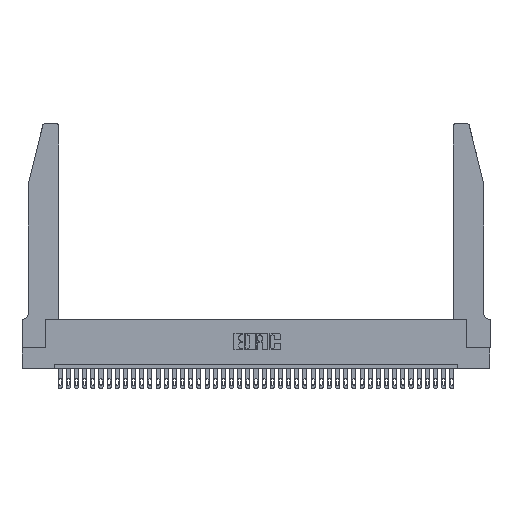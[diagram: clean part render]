
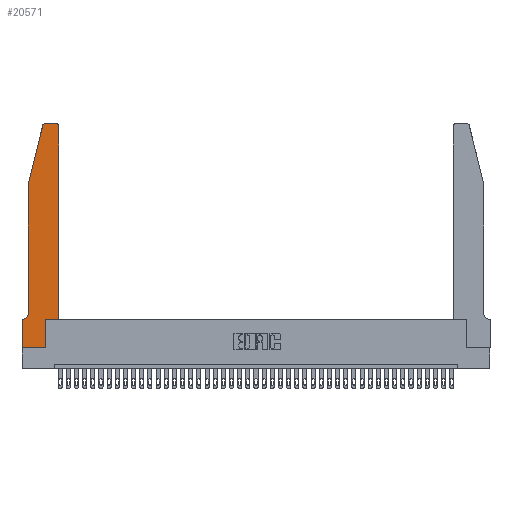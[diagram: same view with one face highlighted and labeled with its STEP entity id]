
A CAD part, top view. The second image highlights one B-rep face of the part: STEP entity #20571.
In plain terms, the highlighted planar face has unit normal (0, 0, 1).
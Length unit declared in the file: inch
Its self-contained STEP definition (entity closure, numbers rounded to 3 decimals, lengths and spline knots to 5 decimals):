
#748 = ORIENTED_EDGE ( 'NONE', *, *, #4426, .T. ) ;
#817 = CARTESIAN_POINT ( 'NONE',  ( 0., 0., 0.37 ) ) ;
#852 = CARTESIAN_POINT ( 'NONE',  ( 0.4505, 0.35, 0.37 ) ) ;
#2289 = EDGE_CURVE ( 'NONE', #5281, #23859, #35067, .T. ) ;
#2867 = CARTESIAN_POINT ( 'NONE',  ( 0.284, 2.75, 0.37 ) ) ;
#3310 = VERTEX_POINT ( 'NONE', #32495 ) ;
#3623 = ORIENTED_EDGE ( 'NONE', *, *, #15255, .T. ) ;
#4426 = EDGE_CURVE ( 'NONE', #23859, #28531, #38317, .T. ) ;
#4523 = ORIENTED_EDGE ( 'NONE', *, *, #11093, .T. ) ;
#4925 = CARTESIAN_POINT ( 'NONE',  ( 0.4505, 0.35, 0.37 ) ) ;
#5281 = VERTEX_POINT ( 'NONE', #11963 ) ;
#5497 = VECTOR ( 'NONE', #39583, 39.37008 ) ;
#5569 = AXIS2_PLACEMENT_3D ( 'NONE', #24513, #27933, #27670 ) ;
#5633 = CARTESIAN_POINT ( 'NONE',  ( 0.4505, 2.72, 0.37 ) ) ;
#5838 = CARTESIAN_POINT ( 'NONE',  ( 0.0055, 0.42, 0.37 ) ) ;
#6523 = CARTESIAN_POINT ( 'NONE',  ( 0.0755, 0.42, 0.37 ) ) ;
#6568 = DIRECTION ( 'NONE',  ( 0., 0., 1. ) ) ;
#6825 = CARTESIAN_POINT ( 'NONE',  ( 0.4205, 2.72, 0.37 ) ) ;
#7433 = EDGE_CURVE ( 'NONE', #28531, #3310, #31796, .T. ) ;
#8090 = DIRECTION ( 'NONE',  ( 1., 0., 0. ) ) ;
#8739 = ORIENTED_EDGE ( 'NONE', *, *, #37533, .T. ) ;
#8813 = ORIENTED_EDGE ( 'NONE', *, *, #30957, .T. ) ;
#8863 = VECTOR ( 'NONE', #28510, 39.37008 ) ;
#8912 = VECTOR ( 'NONE', #32799, 39.37008 ) ;
#9262 = ORIENTED_EDGE ( 'NONE', *, *, #27875, .T. ) ;
#9658 = VECTOR ( 'NONE', #8090, 39.37008 ) ;
#10449 = AXIS2_PLACEMENT_3D ( 'NONE', #5838, #27757, #28027 ) ;
#11093 = EDGE_CURVE ( 'NONE', #25841, #20115, #26158, .T. ) ;
#11632 = EDGE_CURVE ( 'NONE', #16073, #5281, #38795, .T. ) ;
#11963 = CARTESIAN_POINT ( 'NONE',  ( 0., 0.35, 0.37 ) ) ;
#12332 = CARTESIAN_POINT ( 'NONE',  ( 0.0755, 2., 0.37 ) ) ;
#12408 = EDGE_CURVE ( 'NONE', #18849, #21937, #33469, .T. ) ;
#13121 = DIRECTION ( 'NONE',  ( 1., 0., 0. ) ) ;
#13303 = CIRCLE ( 'NONE', #14146, 0.03 ) ;
#14146 = AXIS2_PLACEMENT_3D ( 'NONE', #29347, #29221, #23728 ) ;
#14297 = CARTESIAN_POINT ( 'NONE',  ( 0.0755, 2., 0.37 ) ) ;
#15255 = EDGE_CURVE ( 'NONE', #35445, #38156, #19973, .T. ) ;
#16073 = VERTEX_POINT ( 'NONE', #18164 ) ;
#16090 = DIRECTION ( 'NONE',  ( 0., -1., 0. ) ) ;
#16296 = ORIENTED_EDGE ( 'NONE', *, *, #25361, .T. ) ;
#16523 = LINE ( 'NONE', #4925, #9658 ) ;
#16772 = VECTOR ( 'NONE', #33223, 39.37008 ) ;
#17931 = CIRCLE ( 'NONE', #35897, 0.03 ) ;
#18146 = PLANE ( 'NONE',  #5569 ) ;
#18164 = CARTESIAN_POINT ( 'NONE',  ( 0.0055, 0.35, 0.37 ) ) ;
#18655 = VECTOR ( 'NONE', #13121, 39.37008 ) ;
#18849 = VERTEX_POINT ( 'NONE', #33351 ) ;
#18948 = EDGE_CURVE ( 'NONE', #35115, #16073, #20151, .T. ) ;
#19116 = FACE_OUTER_BOUND ( 'NONE', #30103, .T. ) ;
#19641 = LINE ( 'NONE', #12332, #8863 ) ;
#19654 = CARTESIAN_POINT ( 'NONE',  ( 0., 0., 0.37 ) ) ;
#19973 = LINE ( 'NONE', #38960, #28348 ) ;
#20115 = VERTEX_POINT ( 'NONE', #5633 ) ;
#20151 = CIRCLE ( 'NONE', #10449, 0.07 ) ;
#20350 = CARTESIAN_POINT ( 'NONE',  ( 0.2865, 0., 0.37 ) ) ;
#20452 = CARTESIAN_POINT ( 'NONE',  ( 0.4205, 2.75, 0.37 ) ) ;
#20547 = CARTESIAN_POINT ( 'NONE',  ( 0.4505, 0.35, 0.37 ) ) ;
#20571 = ADVANCED_FACE ( 'NONE', ( #19116 ), #18146, .T. ) ;
#21937 = VERTEX_POINT ( 'NONE', #14297 ) ;
#22474 = ORIENTED_EDGE ( 'NONE', *, *, #18948, .T. ) ;
#23728 = DIRECTION ( 'NONE',  ( 1., 0., 0. ) ) ;
#23859 = VERTEX_POINT ( 'NONE', #817 ) ;
#24513 = CARTESIAN_POINT ( 'NONE',  ( 0., 0.35, 0.37 ) ) ;
#24983 = CARTESIAN_POINT ( 'NONE',  ( 0.2865, 0.35, 0.37 ) ) ;
#25361 = EDGE_CURVE ( 'NONE', #20115, #35445, #17931, .T. ) ;
#25782 = DIRECTION ( 'NONE',  ( 0., 1., 0. ) ) ;
#25841 = VERTEX_POINT ( 'NONE', #852 ) ;
#25962 = DIRECTION ( 'NONE',  ( -1., 0., 0. ) ) ;
#26158 = LINE ( 'NONE', #20547, #16772 ) ;
#26651 = ORIENTED_EDGE ( 'NONE', *, *, #2289, .T. ) ;
#27670 = DIRECTION ( 'NONE',  ( 1., 0., 0. ) ) ;
#27757 = DIRECTION ( 'NONE',  ( 0., 0., -1. ) ) ;
#27875 = EDGE_CURVE ( 'NONE', #38156, #18849, #13303, .T. ) ;
#27933 = DIRECTION ( 'NONE',  ( 0., 0., 1. ) ) ;
#28027 = DIRECTION ( 'NONE',  ( -1., 0., 0. ) ) ;
#28348 = VECTOR ( 'NONE', #25962, 39.37008 ) ;
#28510 = DIRECTION ( 'NONE',  ( 0., -1., 0. ) ) ;
#28531 = VERTEX_POINT ( 'NONE', #20350 ) ;
#29221 = DIRECTION ( 'NONE',  ( 0., 0., 1. ) ) ;
#29347 = CARTESIAN_POINT ( 'NONE',  ( 0.284, 2.72, 0.37 ) ) ;
#30103 = EDGE_LOOP ( 'NONE', ( #3623, #9262, #34498, #8739, #22474, #38598, #26651, #748, #33098, #8813, #4523, #16296 ) ) ;
#30957 = EDGE_CURVE ( 'NONE', #3310, #25841, #16523, .T. ) ;
#31665 = VECTOR ( 'NONE', #16090, 39.37008 ) ;
#31796 = LINE ( 'NONE', #24983, #40139 ) ;
#31961 = CARTESIAN_POINT ( 'NONE',  ( 0., 0., 0.37 ) ) ;
#32495 = CARTESIAN_POINT ( 'NONE',  ( 0.2865, 0.35, 0.37 ) ) ;
#32799 = DIRECTION ( 'NONE',  ( -1., 0., 0. ) ) ;
#33098 = ORIENTED_EDGE ( 'NONE', *, *, #7433, .T. ) ;
#33223 = DIRECTION ( 'NONE',  ( 0., 1., 0. ) ) ;
#33319 = CARTESIAN_POINT ( 'NONE',  ( 0.0755, 2., 0.37 ) ) ;
#33351 = CARTESIAN_POINT ( 'NONE',  ( 0.25487, 2.72718, 0.37 ) ) ;
#33469 = LINE ( 'NONE', #33319, #5497 ) ;
#34498 = ORIENTED_EDGE ( 'NONE', *, *, #12408, .T. ) ;
#34673 = DIRECTION ( 'NONE',  ( 1., 0., 0. ) ) ;
#35067 = LINE ( 'NONE', #19654, #31665 ) ;
#35115 = VERTEX_POINT ( 'NONE', #6523 ) ;
#35126 = CARTESIAN_POINT ( 'NONE',  ( 0.0755, 0.35, 0.37 ) ) ;
#35445 = VERTEX_POINT ( 'NONE', #20452 ) ;
#35897 = AXIS2_PLACEMENT_3D ( 'NONE', #6825, #6568, #34673 ) ;
#37533 = EDGE_CURVE ( 'NONE', #21937, #35115, #19641, .T. ) ;
#38156 = VERTEX_POINT ( 'NONE', #2867 ) ;
#38317 = LINE ( 'NONE', #31961, #18655 ) ;
#38598 = ORIENTED_EDGE ( 'NONE', *, *, #11632, .T. ) ;
#38795 = LINE ( 'NONE', #35126, #8912 ) ;
#38960 = CARTESIAN_POINT ( 'NONE',  ( 0.2605, 2.75, 0.37 ) ) ;
#39583 = DIRECTION ( 'NONE',  ( -0.239, -0.971, 0. ) ) ;
#40139 = VECTOR ( 'NONE', #25782, 39.37008 ) ;
